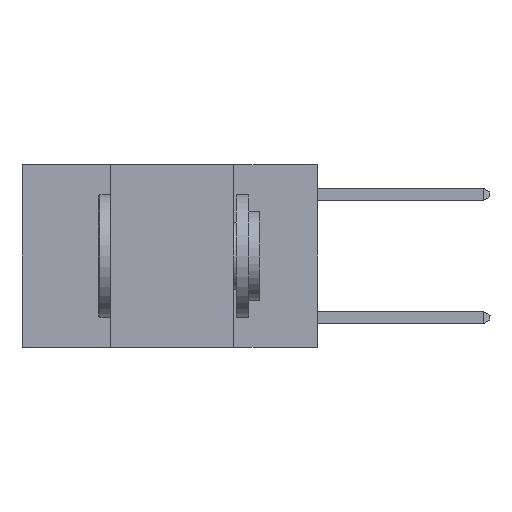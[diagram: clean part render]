
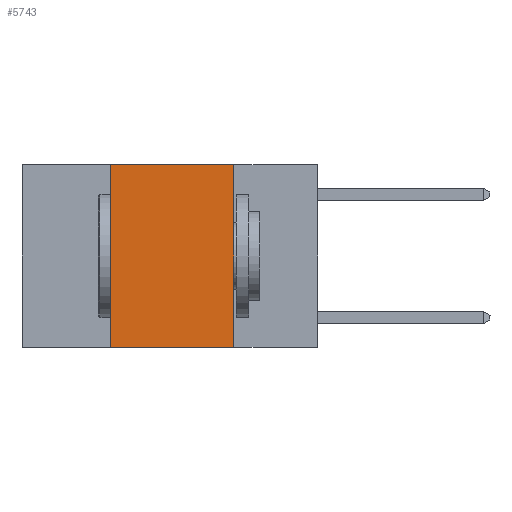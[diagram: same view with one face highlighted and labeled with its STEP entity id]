
A CAD part, left-side view. The second image highlights one B-rep face of the part: STEP entity #5743.
In plain terms, the highlighted planar face has unit normal (-1, 0, 0).
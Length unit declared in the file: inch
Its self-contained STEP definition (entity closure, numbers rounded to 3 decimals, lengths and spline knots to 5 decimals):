
#1664 = DIRECTION ( 'NONE',  ( 0., 0., 1. ) ) ;
#2049 = CARTESIAN_POINT ( 'NONE',  ( 0., 0.6, 0. ) ) ;
#2458 = VECTOR ( 'NONE', #11237, 39.37008 ) ;
#3050 = FACE_OUTER_BOUND ( 'NONE', #17128, .T. ) ;
#3223 = LINE ( 'NONE', #17024, #20768 ) ;
#4300 = DIRECTION ( 'NONE',  ( 1., 0., 0. ) ) ;
#5475 = CARTESIAN_POINT ( 'NONE',  ( 0., 0.42, 0. ) ) ;
#5743 = ADVANCED_FACE ( 'NONE', ( #3050 ), #9435, .F. ) ;
#6016 = ORIENTED_EDGE ( 'NONE', *, *, #11204, .F. ) ;
#6598 = DIRECTION ( 'NONE',  ( 0., 0., -1. ) ) ;
#6917 = ORIENTED_EDGE ( 'NONE', *, *, #7924, .F. ) ;
#7185 = LINE ( 'NONE', #16795, #16280 ) ;
#7788 = EDGE_CURVE ( 'NONE', #14513, #11457, #3223, .T. ) ;
#7924 = EDGE_CURVE ( 'NONE', #11457, #18347, #13494, .T. ) ;
#8361 = VERTEX_POINT ( 'NONE', #9882 ) ;
#8838 = ORIENTED_EDGE ( 'NONE', *, *, #7788, .F. ) ;
#9435 = PLANE ( 'NONE',  #10190 ) ;
#9882 = CARTESIAN_POINT ( 'NONE',  ( 0., 0.17, -0.37 ) ) ;
#10007 = VECTOR ( 'NONE', #14103, 39.37008 ) ;
#10190 = AXIS2_PLACEMENT_3D ( 'NONE', #12875, #4300, #16291 ) ;
#10292 = CARTESIAN_POINT ( 'NONE',  ( 0., 0.42, -0.37 ) ) ;
#10418 = ORIENTED_EDGE ( 'NONE', *, *, #20391, .T. ) ;
#11204 = EDGE_CURVE ( 'NONE', #18347, #8361, #7185, .T. ) ;
#11237 = DIRECTION ( 'NONE',  ( 0., -1., 0. ) ) ;
#11457 = VERTEX_POINT ( 'NONE', #5475 ) ;
#12875 = CARTESIAN_POINT ( 'NONE',  ( 0., 0.6, 0. ) ) ;
#13494 = LINE ( 'NONE', #2049, #10007 ) ;
#14103 = DIRECTION ( 'NONE',  ( 0., -1., 0. ) ) ;
#14513 = VERTEX_POINT ( 'NONE', #10292 ) ;
#16101 = CARTESIAN_POINT ( 'NONE',  ( 0., 0.17, 0. ) ) ;
#16280 = VECTOR ( 'NONE', #6598, 39.37008 ) ;
#16291 = DIRECTION ( 'NONE',  ( 0., 0., -1. ) ) ;
#16403 = CARTESIAN_POINT ( 'NONE',  ( 0., 0.6, -0.37 ) ) ;
#16663 = LINE ( 'NONE', #16403, #2458 ) ;
#16795 = CARTESIAN_POINT ( 'NONE',  ( 0., 0.17, 0. ) ) ;
#17024 = CARTESIAN_POINT ( 'NONE',  ( 0., 0.42, 0. ) ) ;
#17128 = EDGE_LOOP ( 'NONE', ( #6016, #6917, #8838, #10418 ) ) ;
#18347 = VERTEX_POINT ( 'NONE', #16101 ) ;
#20391 = EDGE_CURVE ( 'NONE', #14513, #8361, #16663, .T. ) ;
#20768 = VECTOR ( 'NONE', #1664, 39.37008 ) ;
